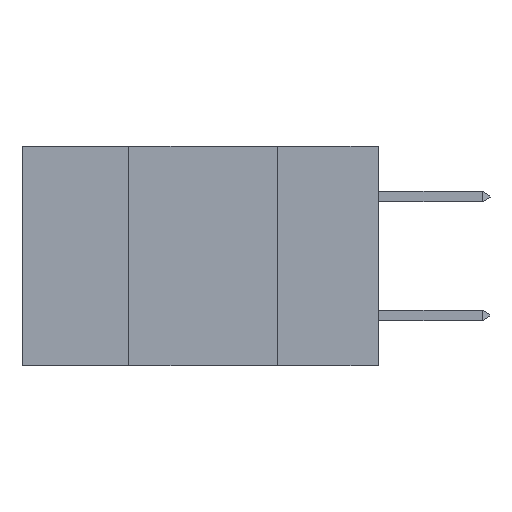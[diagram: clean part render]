
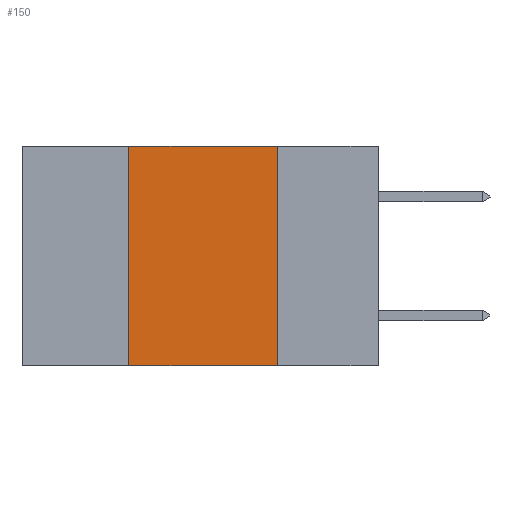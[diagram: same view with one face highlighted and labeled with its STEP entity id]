
A CAD part, left-side view. The second image highlights one B-rep face of the part: STEP entity #150.
In plain terms, the highlighted planar face has unit normal (-1, 0, 0).
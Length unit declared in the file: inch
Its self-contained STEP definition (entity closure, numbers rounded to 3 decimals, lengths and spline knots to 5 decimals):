
#22 = VERTEX_POINT ( 'NONE', #6048 ) ;
#150 = ADVANCED_FACE ( 'NONE', ( #21446 ), #25535, .F. ) ;
#730 = EDGE_CURVE ( 'NONE', #3010, #8491, #14708, .T. ) ;
#3010 = VERTEX_POINT ( 'NONE', #7802 ) ;
#4132 = DIRECTION ( 'NONE',  ( 0., -1., 0. ) ) ;
#4642 = CARTESIAN_POINT ( 'NONE',  ( 0., 0.6, 0. ) ) ;
#5696 = DIRECTION ( 'NONE',  ( 0., 0., -1. ) ) ;
#5740 = DIRECTION ( 'NONE',  ( 1., 0., 0. ) ) ;
#5801 = DIRECTION ( 'NONE',  ( 0., 0., -1. ) ) ;
#6048 = CARTESIAN_POINT ( 'NONE',  ( 0., 0.17, 0. ) ) ;
#7802 = CARTESIAN_POINT ( 'NONE',  ( 0., 0.42, -0.37 ) ) ;
#8491 = VERTEX_POINT ( 'NONE', #16281 ) ;
#8508 = LINE ( 'NONE', #19609, #20837 ) ;
#14017 = EDGE_CURVE ( 'NONE', #22, #8491, #8508, .T. ) ;
#14480 = DIRECTION ( 'NONE',  ( 0., 0., 1. ) ) ;
#14708 = LINE ( 'NONE', #26789, #25520 ) ;
#15291 = VECTOR ( 'NONE', #4132, 39.37008 ) ;
#15788 = CARTESIAN_POINT ( 'NONE',  ( 0., 0.6, 0. ) ) ;
#16153 = ORIENTED_EDGE ( 'NONE', *, *, #14017, .F. ) ;
#16178 = EDGE_CURVE ( 'NONE', #29607, #22, #22140, .T. ) ;
#16281 = CARTESIAN_POINT ( 'NONE',  ( 0., 0.17, -0.37 ) ) ;
#17162 = LINE ( 'NONE', #25982, #28034 ) ;
#18303 = ORIENTED_EDGE ( 'NONE', *, *, #26005, .F. ) ;
#19422 = ORIENTED_EDGE ( 'NONE', *, *, #730, .T. ) ;
#19609 = CARTESIAN_POINT ( 'NONE',  ( 0., 0.17, 0. ) ) ;
#20837 = VECTOR ( 'NONE', #5696, 39.37008 ) ;
#20889 = DIRECTION ( 'NONE',  ( 0., -1., 0. ) ) ;
#21446 = FACE_OUTER_BOUND ( 'NONE', #28027, .T. ) ;
#21536 = CARTESIAN_POINT ( 'NONE',  ( 0., 0.42, 0. ) ) ;
#22140 = LINE ( 'NONE', #15788, #15291 ) ;
#25460 = AXIS2_PLACEMENT_3D ( 'NONE', #4642, #5740, #5801 ) ;
#25520 = VECTOR ( 'NONE', #20889, 39.37008 ) ;
#25535 = PLANE ( 'NONE',  #25460 ) ;
#25982 = CARTESIAN_POINT ( 'NONE',  ( 0., 0.42, 0. ) ) ;
#26005 = EDGE_CURVE ( 'NONE', #3010, #29607, #17162, .T. ) ;
#26789 = CARTESIAN_POINT ( 'NONE',  ( 0., 0.6, -0.37 ) ) ;
#28027 = EDGE_LOOP ( 'NONE', ( #16153, #29186, #18303, #19422 ) ) ;
#28034 = VECTOR ( 'NONE', #14480, 39.37008 ) ;
#29186 = ORIENTED_EDGE ( 'NONE', *, *, #16178, .F. ) ;
#29607 = VERTEX_POINT ( 'NONE', #21536 ) ;
